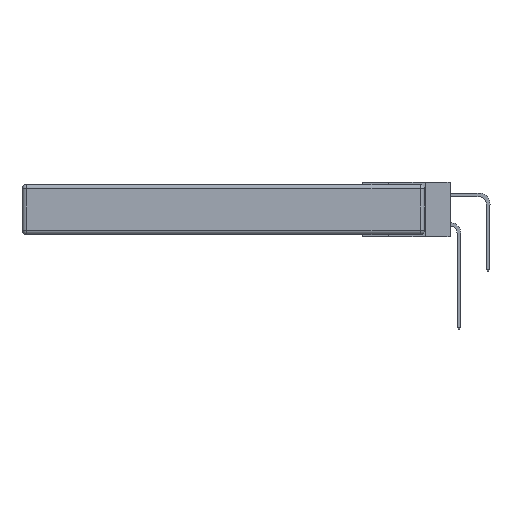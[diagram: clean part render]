
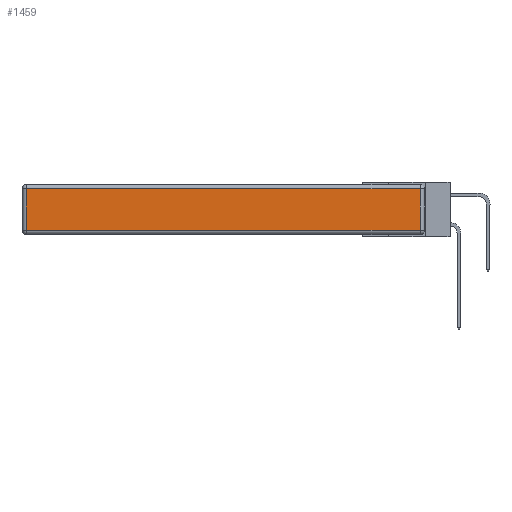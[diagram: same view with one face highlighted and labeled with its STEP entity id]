
A CAD part, left-side view. The second image highlights one B-rep face of the part: STEP entity #1459.
In plain terms, the highlighted planar face has unit normal (-1, 0, 0).
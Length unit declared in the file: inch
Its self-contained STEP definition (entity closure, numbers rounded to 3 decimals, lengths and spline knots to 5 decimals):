
#46 = CARTESIAN_POINT ( 'NONE',  ( 0., 0., -0.313 ) ) ;
#312 = EDGE_CURVE ( 'NONE', #5962, #14754, #14558, .T. ) ;
#976 = ORIENTED_EDGE ( 'NONE', *, *, #3960, .T. ) ;
#1224 = DIRECTION ( 'NONE',  ( 0., 0., 1. ) ) ;
#1290 = CARTESIAN_POINT ( 'NONE',  ( 0., 2.72, -0.343 ) ) ;
#1459 = ADVANCED_FACE ( 'NONE', ( #11136 ), #3442, .T. ) ;
#1920 = LINE ( 'NONE', #46, #8542 ) ;
#2138 = VECTOR ( 'NONE', #15162, 39.37008 ) ;
#2306 = CARTESIAN_POINT ( 'NONE',  ( 0., 0., -0.343 ) ) ;
#3440 = CARTESIAN_POINT ( 'NONE',  ( 0., 0.03, -0.343 ) ) ;
#3442 = PLANE ( 'NONE',  #10814 ) ;
#3960 = EDGE_CURVE ( 'NONE', #14469, #9689, #14320, .T. ) ;
#4672 = DIRECTION ( 'NONE',  ( -1., 0., 0. ) ) ;
#5228 = VECTOR ( 'NONE', #14648, 39.37008 ) ;
#5962 = VERTEX_POINT ( 'NONE', #6391 ) ;
#6119 = ORIENTED_EDGE ( 'NONE', *, *, #9555, .T. ) ;
#6141 = LINE ( 'NONE', #13437, #5228 ) ;
#6194 = DIRECTION ( 'NONE',  ( 0., 0., -1. ) ) ;
#6391 = CARTESIAN_POINT ( 'NONE',  ( 0., 2.72, -0.03 ) ) ;
#7741 = VECTOR ( 'NONE', #6194, 39.37008 ) ;
#8542 = VECTOR ( 'NONE', #14143, 39.37008 ) ;
#9367 = CARTESIAN_POINT ( 'NONE',  ( 0., 0.03, -0.03 ) ) ;
#9555 = EDGE_CURVE ( 'NONE', #14754, #14469, #1920, .T. ) ;
#9689 = VERTEX_POINT ( 'NONE', #9367 ) ;
#10814 = AXIS2_PLACEMENT_3D ( 'NONE', #2306, #4672, #1224 ) ;
#10988 = ORIENTED_EDGE ( 'NONE', *, *, #312, .T. ) ;
#11136 = FACE_OUTER_BOUND ( 'NONE', #14987, .T. ) ;
#12683 = CARTESIAN_POINT ( 'NONE',  ( 0., 0.03, -0.313 ) ) ;
#13117 = CARTESIAN_POINT ( 'NONE',  ( 0., 2.72, -0.313 ) ) ;
#13437 = CARTESIAN_POINT ( 'NONE',  ( 0., 2.75, -0.03 ) ) ;
#13469 = ORIENTED_EDGE ( 'NONE', *, *, #14348, .T. ) ;
#14143 = DIRECTION ( 'NONE',  ( 0., -1., 0. ) ) ;
#14320 = LINE ( 'NONE', #3440, #2138 ) ;
#14348 = EDGE_CURVE ( 'NONE', #9689, #5962, #6141, .T. ) ;
#14469 = VERTEX_POINT ( 'NONE', #12683 ) ;
#14558 = LINE ( 'NONE', #1290, #7741 ) ;
#14648 = DIRECTION ( 'NONE',  ( 0., 1., 0. ) ) ;
#14754 = VERTEX_POINT ( 'NONE', #13117 ) ;
#14987 = EDGE_LOOP ( 'NONE', ( #6119, #976, #13469, #10988 ) ) ;
#15162 = DIRECTION ( 'NONE',  ( 0., 0., 1. ) ) ;
